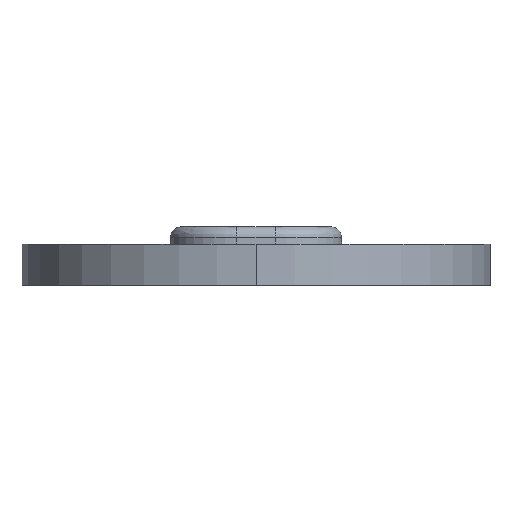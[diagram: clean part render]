
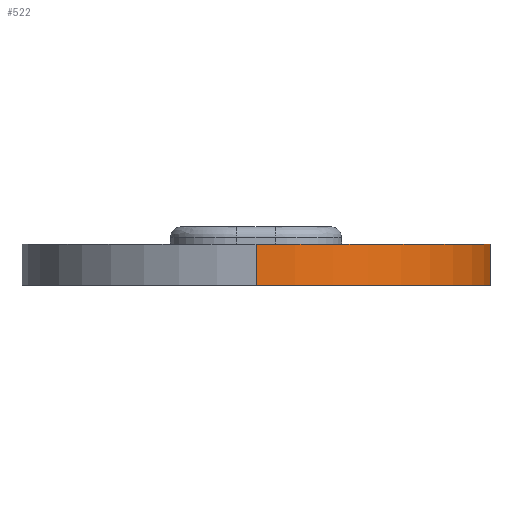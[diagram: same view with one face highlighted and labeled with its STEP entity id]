
A CAD part, left-side view. The second image highlights one B-rep face of the part: STEP entity #522.
In plain terms, the highlighted cylindrical face has radius 17.361 mm (diameter 34.722 mm), a partial arc.
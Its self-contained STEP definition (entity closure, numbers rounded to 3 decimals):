
#15 = ORIENTED_EDGE ( 'NONE', *, *, #661, .T. ) ;
#23 = VERTEX_POINT ( 'NONE', #570 ) ;
#31 = VERTEX_POINT ( 'NONE', #106 ) ;
#40 = ORIENTED_EDGE ( 'NONE', *, *, #667, .T. ) ;
#54 = ORIENTED_EDGE ( 'NONE', *, *, #662, .T. ) ;
#93 = ORIENTED_EDGE ( 'NONE', *, *, #670, .T. ) ;
#106 = CARTESIAN_POINT ( 'NONE',  ( -11.504, -16.775, 0. ) ) ;
#202 = EDGE_LOOP ( 'NONE', ( #93, #40, #54, #15 ) ) ;
#256 = DIRECTION ( 'NONE',  ( 0., 0., -1. ) ) ;
#288 = VERTEX_POINT ( 'NONE', #633 ) ;
#301 = FACE_OUTER_BOUND ( 'NONE', #202, .T. ) ;
#350 = CIRCLE ( 'NONE', #612, 17.361 ) ;
#351 = CARTESIAN_POINT ( 'NONE',  ( -11.504, -16.775, 3.035 ) ) ;
#355 = DIRECTION ( 'NONE',  ( 0., 0., 1. ) ) ;
#363 = CARTESIAN_POINT ( 'NONE',  ( -33.337, 0., 3.035 ) ) ;
#366 = DIRECTION ( 'NONE',  ( 0., 0., -1. ) ) ;
#368 = CARTESIAN_POINT ( 'NONE',  ( -15.977, 0., 0. ) ) ;
#372 = DIRECTION ( 'NONE',  ( 0., 0., 1. ) ) ;
#374 = DIRECTION ( 'NONE',  ( -1., 0., 0. ) ) ;
#396 = VECTOR ( 'NONE', #355, 1000. ) ;
#397 = LINE ( 'NONE', #363, #888 ) ;
#398 = LINE ( 'NONE', #351, #396 ) ;
#402 = CARTESIAN_POINT ( 'NONE',  ( -11.504, -16.775, 3.035 ) ) ;
#420 = CARTESIAN_POINT ( 'NONE',  ( -15.977, 0., 3.035 ) ) ;
#430 = DIRECTION ( 'NONE',  ( 0., 0., -1. ) ) ;
#461 = DIRECTION ( 'NONE',  ( -1., 0., 0. ) ) ;
#463 = DIRECTION ( 'NONE',  ( -1., 0., 0. ) ) ;
#522 = ADVANCED_FACE ( 'NONE', ( #301 ), #774, .T. ) ;
#570 = CARTESIAN_POINT ( 'NONE',  ( -33.337, 0., 0. ) ) ;
#575 = VERTEX_POINT ( 'NONE', #402 ) ;
#606 = AXIS2_PLACEMENT_3D ( 'NONE', #420, #430, #463 ) ;
#612 = AXIS2_PLACEMENT_3D ( 'NONE', #368, #372, #374 ) ;
#622 = AXIS2_PLACEMENT_3D ( 'NONE', #731, #256, #461 ) ;
#633 = CARTESIAN_POINT ( 'NONE',  ( -33.337, 0., 3.035 ) ) ;
#661 = EDGE_CURVE ( 'NONE', #31, #575, #398, .T. ) ;
#662 = EDGE_CURVE ( 'NONE', #23, #31, #350, .T. ) ;
#667 = EDGE_CURVE ( 'NONE', #288, #23, #397, .T. ) ;
#670 = EDGE_CURVE ( 'NONE', #575, #288, #871, .T. ) ;
#731 = CARTESIAN_POINT ( 'NONE',  ( -15.977, 0., 3.035 ) ) ;
#774 = CYLINDRICAL_SURFACE ( 'NONE', #622, 17.361 ) ;
#871 = CIRCLE ( 'NONE', #606, 17.361 ) ;
#888 = VECTOR ( 'NONE', #366, 1000. ) ;
